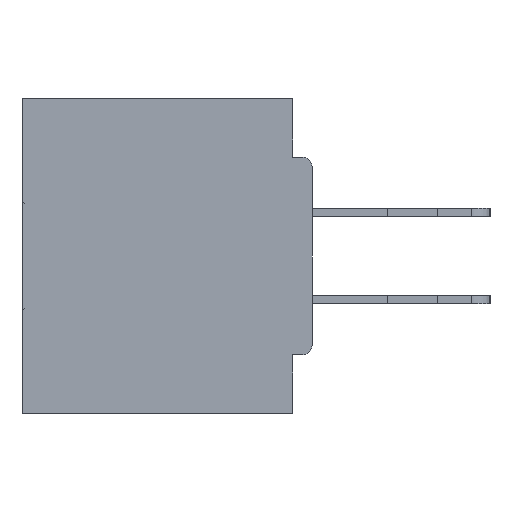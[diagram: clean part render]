
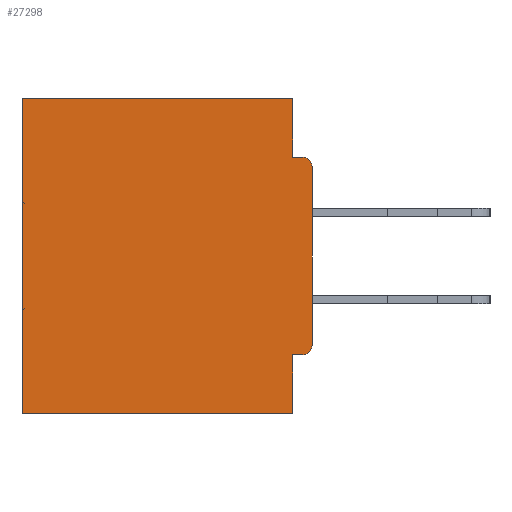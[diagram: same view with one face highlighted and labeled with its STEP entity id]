
A CAD part, left-side view. The second image highlights one B-rep face of the part: STEP entity #27298.
In plain terms, the highlighted planar face has unit normal (-1, 0, 0).
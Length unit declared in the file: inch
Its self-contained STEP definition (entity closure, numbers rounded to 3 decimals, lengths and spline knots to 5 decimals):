
#2289 = VERTEX_POINT ( 'NONE', #40728 ) ;
#2777 = AXIS2_PLACEMENT_3D ( 'NONE', #36815, #23361, #19679 ) ;
#3240 = CARTESIAN_POINT ( 'NONE',  ( 0.298, 0.46, -0.5 ) ) ;
#4040 = VECTOR ( 'NONE', #14313, 39.37008 ) ;
#4144 = FACE_OUTER_BOUND ( 'NONE', #7284, .T. ) ;
#4180 = VERTEX_POINT ( 'NONE', #19315 ) ;
#4306 = CARTESIAN_POINT ( 'NONE',  ( 0.298, 0., -0.0935 ) ) ;
#6415 = DIRECTION ( 'NONE',  ( 0., 0., -1. ) ) ;
#6799 = ORIENTED_EDGE ( 'NONE', *, *, #24990, .T. ) ;
#7164 = LINE ( 'NONE', #33916, #23613 ) ;
#7240 = VECTOR ( 'NONE', #44231, 39.37008 ) ;
#7284 = EDGE_LOOP ( 'NONE', ( #13068, #39949, #39542, #35616, #33977, #28904, #27835, #29041, #6799, #7401 ) ) ;
#7401 = ORIENTED_EDGE ( 'NONE', *, *, #28379, .F. ) ;
#7811 = DIRECTION ( 'NONE',  ( 0., -1., 0. ) ) ;
#8695 = DIRECTION ( 'NONE',  ( -1., 0., 0. ) ) ;
#9182 = EDGE_CURVE ( 'NONE', #29582, #31976, #27164, .T. ) ;
#9835 = VECTOR ( 'NONE', #7811, 39.37008 ) ;
#11162 = CARTESIAN_POINT ( 'NONE',  ( 0.298, 0.031, -0.5 ) ) ;
#11996 = DIRECTION ( 'NONE',  ( 0., 0., -1. ) ) ;
#12030 = CIRCLE ( 'NONE', #36248, 0.015 ) ;
#12160 = CARTESIAN_POINT ( 'NONE',  ( 0.298, 0., -0.5 ) ) ;
#13068 = ORIENTED_EDGE ( 'NONE', *, *, #9182, .T. ) ;
#14313 = DIRECTION ( 'NONE',  ( 0., 1., 0. ) ) ;
#14858 = EDGE_CURVE ( 'NONE', #34145, #29552, #33068, .T. ) ;
#16439 = LINE ( 'NONE', #18902, #17491 ) ;
#17491 = VECTOR ( 'NONE', #11996, 39.37008 ) ;
#17697 = VECTOR ( 'NONE', #17719, 39.37008 ) ;
#17719 = DIRECTION ( 'NONE',  ( 0., 0., -1. ) ) ;
#18870 = VERTEX_POINT ( 'NONE', #25614 ) ;
#18902 = CARTESIAN_POINT ( 'NONE',  ( 0.298, 0.46, 0. ) ) ;
#19315 = CARTESIAN_POINT ( 'NONE',  ( 0.298, 0.031, 0. ) ) ;
#19679 = DIRECTION ( 'NONE',  ( 0., 0., -1. ) ) ;
#19929 = EDGE_CURVE ( 'NONE', #2289, #18870, #33028, .T. ) ;
#19978 = PLANE ( 'NONE',  #2777 ) ;
#20114 = DIRECTION ( 'NONE',  ( 0., 1., 0. ) ) ;
#20475 = LINE ( 'NONE', #11162, #17697 ) ;
#20741 = CARTESIAN_POINT ( 'NONE',  ( 0.298, 0.031, -0.5 ) ) ;
#22167 = CARTESIAN_POINT ( 'NONE',  ( 0.298, 0.015, -0.1085 ) ) ;
#23361 = DIRECTION ( 'NONE',  ( 1., 0., 0. ) ) ;
#23487 = CARTESIAN_POINT ( 'NONE',  ( 0.298, 0.015, -0.0935 ) ) ;
#23613 = VECTOR ( 'NONE', #34080, 39.37008 ) ;
#23760 = VECTOR ( 'NONE', #6415, 39.37008 ) ;
#24873 = EDGE_CURVE ( 'NONE', #42888, #31976, #32820, .T. ) ;
#24990 = EDGE_CURVE ( 'NONE', #2289, #37966, #12030, .T. ) ;
#25614 = CARTESIAN_POINT ( 'NONE',  ( 0.298, 0.031, -0.4065 ) ) ;
#26402 = AXIS2_PLACEMENT_3D ( 'NONE', #22167, #8695, #33015 ) ;
#26748 = DIRECTION ( 'NONE',  ( -1., 0., 0. ) ) ;
#27164 = CIRCLE ( 'NONE', #26402, 0.015 ) ;
#27298 = ADVANCED_FACE ( 'NONE', ( #4144 ), #19978, .F. ) ;
#27558 = VECTOR ( 'NONE', #20114, 39.37008 ) ;
#27585 = VERTEX_POINT ( 'NONE', #31396 ) ;
#27648 = CARTESIAN_POINT ( 'NONE',  ( 0.298, 0., -0.1085 ) ) ;
#27835 = ORIENTED_EDGE ( 'NONE', *, *, #39566, .F. ) ;
#27909 = CARTESIAN_POINT ( 'NONE',  ( 0.298, 0., -0.4065 ) ) ;
#28379 = EDGE_CURVE ( 'NONE', #29582, #37966, #40124, .T. ) ;
#28898 = EDGE_CURVE ( 'NONE', #4180, #42888, #43301, .T. ) ;
#28904 = ORIENTED_EDGE ( 'NONE', *, *, #14858, .F. ) ;
#29041 = ORIENTED_EDGE ( 'NONE', *, *, #19929, .F. ) ;
#29552 = VERTEX_POINT ( 'NONE', #3240 ) ;
#29582 = VERTEX_POINT ( 'NONE', #27648 ) ;
#31396 = CARTESIAN_POINT ( 'NONE',  ( 0.298, 0.46, 0. ) ) ;
#31880 = EDGE_CURVE ( 'NONE', #27585, #29552, #16439, .T. ) ;
#31976 = VERTEX_POINT ( 'NONE', #23487 ) ;
#32820 = LINE ( 'NONE', #4306, #9835 ) ;
#33015 = DIRECTION ( 'NONE',  ( 0., 0., -1. ) ) ;
#33028 = LINE ( 'NONE', #27909, #4040 ) ;
#33068 = LINE ( 'NONE', #12160, #27558 ) ;
#33737 = CARTESIAN_POINT ( 'NONE',  ( 0.298, 0.031, -0.5 ) ) ;
#33916 = CARTESIAN_POINT ( 'NONE',  ( 0.298, 0., 0. ) ) ;
#33977 = ORIENTED_EDGE ( 'NONE', *, *, #31880, .T. ) ;
#34040 = EDGE_CURVE ( 'NONE', #4180, #27585, #7164, .T. ) ;
#34080 = DIRECTION ( 'NONE',  ( 0., 1., 0. ) ) ;
#34145 = VERTEX_POINT ( 'NONE', #20741 ) ;
#34798 = CARTESIAN_POINT ( 'NONE',  ( 0.298, 0., 0. ) ) ;
#35616 = ORIENTED_EDGE ( 'NONE', *, *, #34040, .T. ) ;
#36248 = AXIS2_PLACEMENT_3D ( 'NONE', #44007, #26748, #37330 ) ;
#36815 = CARTESIAN_POINT ( 'NONE',  ( 0.298, 0., 0. ) ) ;
#37330 = DIRECTION ( 'NONE',  ( 0., 0., -1. ) ) ;
#37878 = CARTESIAN_POINT ( 'NONE',  ( 0.298, 0., -0.3915 ) ) ;
#37966 = VERTEX_POINT ( 'NONE', #37878 ) ;
#38872 = CARTESIAN_POINT ( 'NONE',  ( 0.298, 0.031, -0.0935 ) ) ;
#39542 = ORIENTED_EDGE ( 'NONE', *, *, #28898, .F. ) ;
#39566 = EDGE_CURVE ( 'NONE', #18870, #34145, #20475, .T. ) ;
#39949 = ORIENTED_EDGE ( 'NONE', *, *, #24873, .F. ) ;
#40124 = LINE ( 'NONE', #34798, #23760 ) ;
#40728 = CARTESIAN_POINT ( 'NONE',  ( 0.298, 0.015, -0.4065 ) ) ;
#42888 = VERTEX_POINT ( 'NONE', #38872 ) ;
#43301 = LINE ( 'NONE', #33737, #7240 ) ;
#44007 = CARTESIAN_POINT ( 'NONE',  ( 0.298, 0.015, -0.3915 ) ) ;
#44231 = DIRECTION ( 'NONE',  ( 0., 0., -1. ) ) ;
